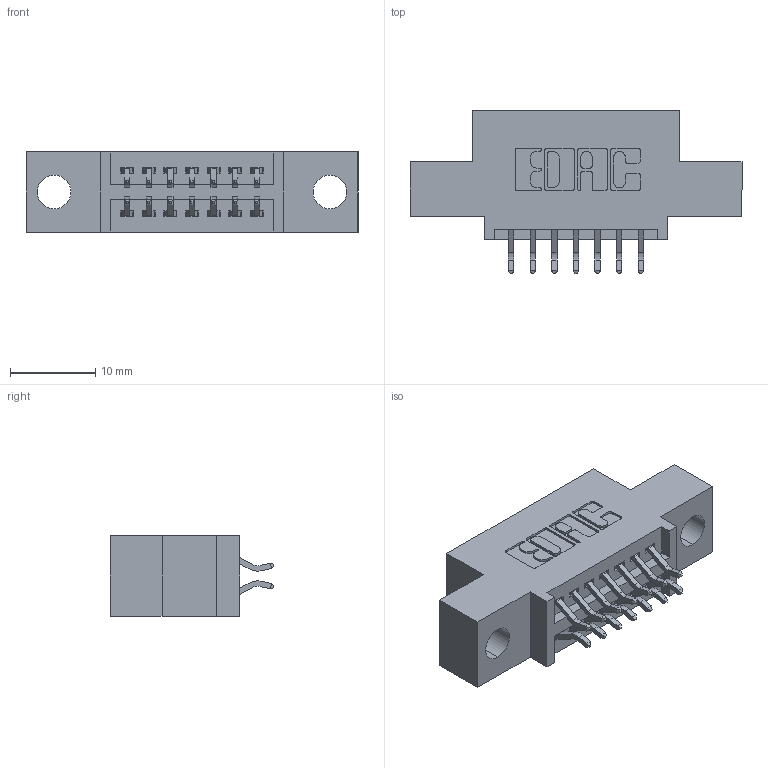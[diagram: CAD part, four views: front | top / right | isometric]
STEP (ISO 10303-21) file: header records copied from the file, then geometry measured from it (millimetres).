
FILE_DESCRIPTION (( 'STEP AP203' ), '1' );
FILE_NAME ('395-014-556-504.STEP', '2021-06-14T18:03:21', ( '' ), ( '' ), 'SwSTEP 2.0', 'SolidWorks 2020', '' );
FILE_SCHEMA (( 'CONFIG_CONTROL_DESIGN' ));
Length unit declared in the file: inch
Products named in the file (3): 345 Part_0.110 Offset - 0.156 Dia-TI; 345-292-001_556 Tail; 395-014-556-504
Assembly tree (15 placements, depth 2):
  395-014-556-504
    345 Part_0.110 Offset - 0.156 Dia-TI
    345-292-001_556 Tail  x14
Bounding box: 38.99 x 19.24 x 9.4 mm (x, y, z)
Volume: 3282.7 mm3; surface area: 4106.6 mm2
Topology: 15 solids, 15 shells, 928 faces, 2727 edges, 1798 vertices
Faces by surface type: plane 616, cylinder 312
Entity records: 10975 total; most frequent: CARTESIAN_POINT 1894, ORIENTED_EDGE 1814, DIRECTION 1699, EDGE_CURVE 907, LINE 739, VECTOR 739, VERTEX_POINT 602, AXIS2_PLACEMENT_3D 480
